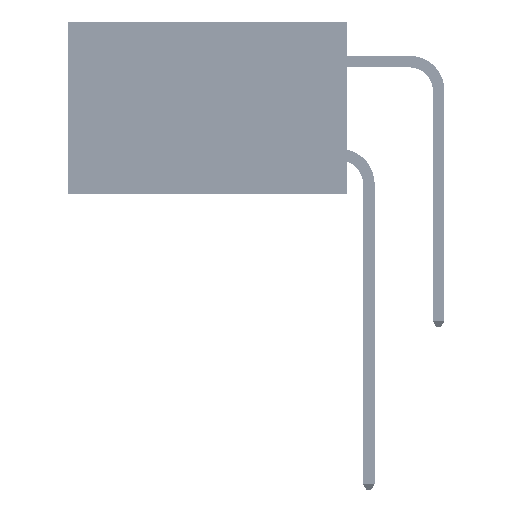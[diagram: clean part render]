
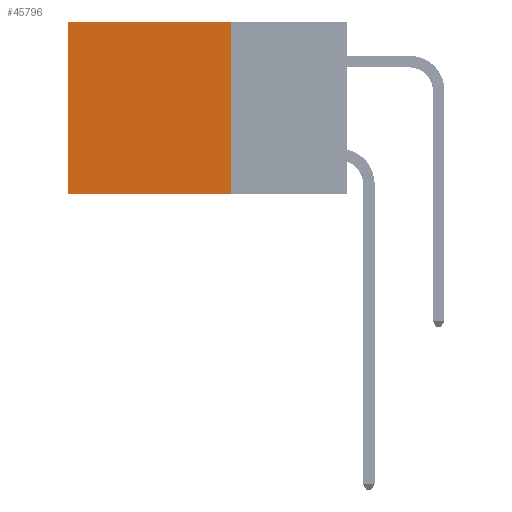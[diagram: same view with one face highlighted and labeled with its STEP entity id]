
A CAD part, left-side view. The second image highlights one B-rep face of the part: STEP entity #45796.
In plain terms, the highlighted planar face has unit normal (-1, 0, 0).
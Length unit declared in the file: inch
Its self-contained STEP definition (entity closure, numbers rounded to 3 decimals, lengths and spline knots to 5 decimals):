
#5283 = DIRECTION ( 'NONE',  ( 0., 1., 0. ) ) ;
#6772 = ORIENTED_EDGE ( 'NONE', *, *, #29529, .F. ) ;
#7592 = DIRECTION ( 'NONE',  ( 0., 0., -1. ) ) ;
#8827 = DIRECTION ( 'NONE',  ( 0., 0., -1. ) ) ;
#10509 = VECTOR ( 'NONE', #8827, 39.37008 ) ;
#11943 = VECTOR ( 'NONE', #24274, 39.37008 ) ;
#11957 = VERTEX_POINT ( 'NONE', #17163 ) ;
#13916 = DIRECTION ( 'NONE',  ( 0., 0., -1. ) ) ;
#14197 = VERTEX_POINT ( 'NONE', #28642 ) ;
#17163 = CARTESIAN_POINT ( 'NONE',  ( 0.2875, 0.25, -0.37 ) ) ;
#17748 = AXIS2_PLACEMENT_3D ( 'NONE', #28486, #20680, #7592 ) ;
#19082 = EDGE_CURVE ( 'NONE', #46241, #39992, #41555, .T. ) ;
#20680 = DIRECTION ( 'NONE',  ( 1., 0., 0. ) ) ;
#21469 = LINE ( 'NONE', #35908, #25302 ) ;
#21899 = VECTOR ( 'NONE', #5283, 39.37008 ) ;
#21955 = CARTESIAN_POINT ( 'NONE',  ( 0.2875, 0.25, 0. ) ) ;
#23129 = ORIENTED_EDGE ( 'NONE', *, *, #45041, .T. ) ;
#24274 = DIRECTION ( 'NONE',  ( 0., 1., 0. ) ) ;
#25302 = VECTOR ( 'NONE', #13916, 39.37008 ) ;
#26585 = CARTESIAN_POINT ( 'NONE',  ( 0.2875, 0.25, -0.37 ) ) ;
#28312 = EDGE_CURVE ( 'NONE', #11957, #14197, #37212, .T. ) ;
#28460 = ORIENTED_EDGE ( 'NONE', *, *, #28312, .F. ) ;
#28486 = CARTESIAN_POINT ( 'NONE',  ( 0.2875, 0.25, 0. ) ) ;
#28642 = CARTESIAN_POINT ( 'NONE',  ( 0.2875, 0.6, -0.37 ) ) ;
#29529 = EDGE_CURVE ( 'NONE', #46241, #11957, #34374, .T. ) ;
#33391 = EDGE_LOOP ( 'NONE', ( #23129, #28460, #6772, #33831 ) ) ;
#33831 = ORIENTED_EDGE ( 'NONE', *, *, #19082, .T. ) ;
#34374 = LINE ( 'NONE', #44562, #10509 ) ;
#35908 = CARTESIAN_POINT ( 'NONE',  ( 0.2875, 0.6, 0. ) ) ;
#37212 = LINE ( 'NONE', #26585, #21899 ) ;
#39992 = VERTEX_POINT ( 'NONE', #41088 ) ;
#39999 = FACE_OUTER_BOUND ( 'NONE', #33391, .T. ) ;
#41088 = CARTESIAN_POINT ( 'NONE',  ( 0.2875, 0.6, 0. ) ) ;
#41555 = LINE ( 'NONE', #45571, #11943 ) ;
#42470 = PLANE ( 'NONE',  #17748 ) ;
#44562 = CARTESIAN_POINT ( 'NONE',  ( 0.2875, 0.25, 0. ) ) ;
#45041 = EDGE_CURVE ( 'NONE', #39992, #14197, #21469, .T. ) ;
#45571 = CARTESIAN_POINT ( 'NONE',  ( 0.2875, 0.25, 0. ) ) ;
#45796 = ADVANCED_FACE ( 'NONE', ( #39999 ), #42470, .F. ) ;
#46241 = VERTEX_POINT ( 'NONE', #21955 ) ;
